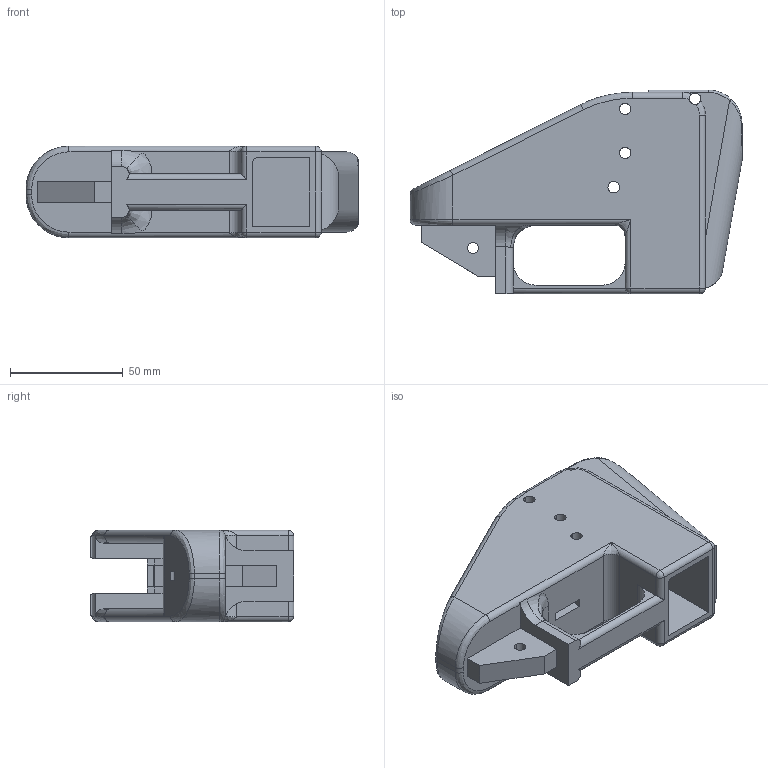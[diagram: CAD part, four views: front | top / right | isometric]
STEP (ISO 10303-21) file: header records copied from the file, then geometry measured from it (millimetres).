
FILE_DESCRIPTION (( 'STEP AP214' ), '1' );
FILE_NAME ('liberatorglockframe.STEP', '2013-06-29T18:32:45', ( '' ), ( '' ), 'SwSTEP 2.0', 'SolidWorks 2012', '' );
FILE_SCHEMA (( 'AUTOMOTIVE_DESIGN' ));
Length unit declared in the file: millimetre
Products named in the file (1): liberatorglockframe
Bounding box: 147.19 x 90.28 x 40.64 mm (x, y, z)
Volume: 203234.8 mm3; surface area: 51063.4 mm2
Topology: 2 solids, 2 shells, 191 faces, 512 edges, 314 vertices
Faces by surface type: plane 86, cylinder 71, bspline 26, sphere 4, cone 2, torus 2
Entity records: 7011 total; most frequent: CARTESIAN_POINT 2370, ORIENTED_EDGE 1012, DIRECTION 904, EDGE_CURVE 506, VERTEX_POINT 314, AXIS2_PLACEMENT_3D 302, LINE 300, VECTOR 300
